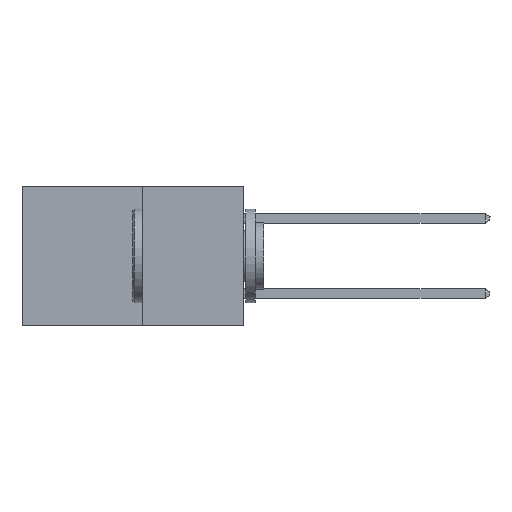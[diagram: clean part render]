
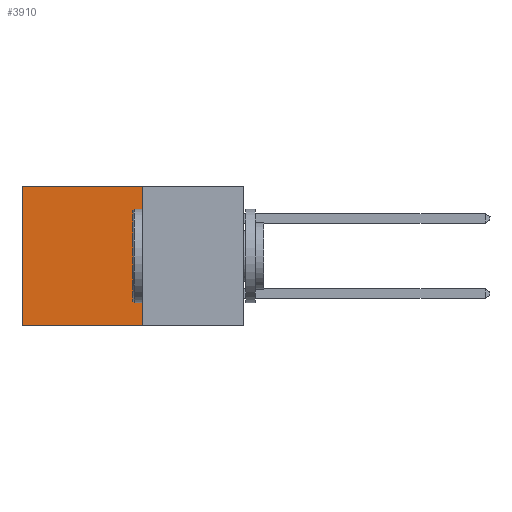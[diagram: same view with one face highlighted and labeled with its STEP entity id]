
A CAD part, left-side view. The second image highlights one B-rep face of the part: STEP entity #3910.
In plain terms, the highlighted planar face has unit normal (-1, 0, 0).
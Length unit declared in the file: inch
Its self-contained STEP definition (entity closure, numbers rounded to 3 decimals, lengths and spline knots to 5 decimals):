
#175 = CARTESIAN_POINT ( 'NONE',  ( 0.277, 0.27, 0. ) ) ;
#395 = DIRECTION ( 'NONE',  ( 0., 1., 0. ) ) ;
#474 = CARTESIAN_POINT ( 'NONE',  ( 0.277, 0.27, 0. ) ) ;
#619 = CARTESIAN_POINT ( 'NONE',  ( 0.277, 0.27, -0.37 ) ) ;
#955 = AXIS2_PLACEMENT_3D ( 'NONE', #7053, #5009, #8291 ) ;
#1451 = CARTESIAN_POINT ( 'NONE',  ( 0.277, 0.59, -0.37 ) ) ;
#1738 = FACE_OUTER_BOUND ( 'NONE', #16087, .T. ) ;
#2416 = LINE ( 'NONE', #1451, #15919 ) ;
#2651 = VERTEX_POINT ( 'NONE', #11530 ) ;
#3036 = VECTOR ( 'NONE', #9922, 39.37008 ) ;
#3564 = LINE ( 'NONE', #5304, #13723 ) ;
#3910 = ADVANCED_FACE ( 'NONE', ( #1738 ), #11478, .F. ) ;
#4383 = EDGE_CURVE ( 'NONE', #5395, #2651, #8872, .T. ) ;
#5009 = DIRECTION ( 'NONE',  ( 1., 0., 0. ) ) ;
#5304 = CARTESIAN_POINT ( 'NONE',  ( 0.277, 0.27, -0.37 ) ) ;
#5395 = VERTEX_POINT ( 'NONE', #175 ) ;
#5703 = VECTOR ( 'NONE', #395, 39.37008 ) ;
#5876 = ORIENTED_EDGE ( 'NONE', *, *, #15933, .T. ) ;
#6357 = ORIENTED_EDGE ( 'NONE', *, *, #16111, .F. ) ;
#6685 = DIRECTION ( 'NONE',  ( 0., 1., 0. ) ) ;
#7053 = CARTESIAN_POINT ( 'NONE',  ( 0.277, 0.27, -0.37 ) ) ;
#7265 = ORIENTED_EDGE ( 'NONE', *, *, #8076, .F. ) ;
#7352 = ORIENTED_EDGE ( 'NONE', *, *, #4383, .T. ) ;
#8076 = EDGE_CURVE ( 'NONE', #10252, #13035, #3564, .T. ) ;
#8291 = DIRECTION ( 'NONE',  ( 0., 0., -1. ) ) ;
#8417 = CARTESIAN_POINT ( 'NONE',  ( 0.277, 0.59, -0.37 ) ) ;
#8872 = LINE ( 'NONE', #474, #5703 ) ;
#9760 = LINE ( 'NONE', #619, #3036 ) ;
#9922 = DIRECTION ( 'NONE',  ( 0., 0., -1. ) ) ;
#10252 = VERTEX_POINT ( 'NONE', #10844 ) ;
#10844 = CARTESIAN_POINT ( 'NONE',  ( 0.277, 0.27, -0.37 ) ) ;
#11478 = PLANE ( 'NONE',  #955 ) ;
#11530 = CARTESIAN_POINT ( 'NONE',  ( 0.277, 0.59, 0. ) ) ;
#13035 = VERTEX_POINT ( 'NONE', #8417 ) ;
#13723 = VECTOR ( 'NONE', #6685, 39.37008 ) ;
#14617 = DIRECTION ( 'NONE',  ( 0., 0., -1. ) ) ;
#15919 = VECTOR ( 'NONE', #14617, 39.37008 ) ;
#15933 = EDGE_CURVE ( 'NONE', #2651, #13035, #2416, .T. ) ;
#16087 = EDGE_LOOP ( 'NONE', ( #5876, #7265, #6357, #7352 ) ) ;
#16111 = EDGE_CURVE ( 'NONE', #5395, #10252, #9760, .T. ) ;
